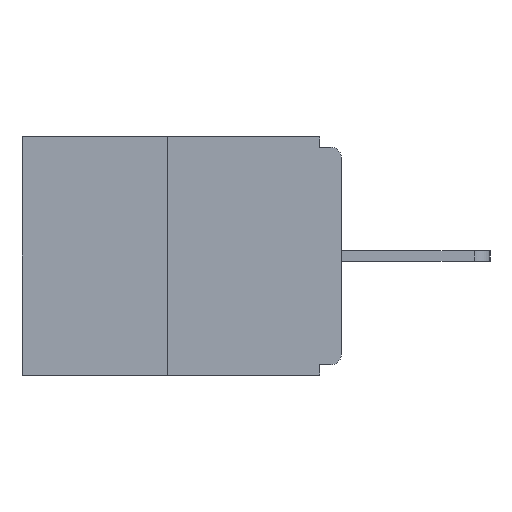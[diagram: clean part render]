
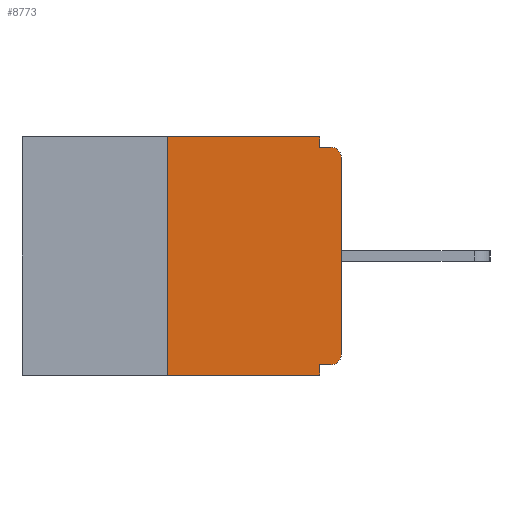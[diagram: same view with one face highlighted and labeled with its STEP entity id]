
A CAD part, left-side view. The second image highlights one B-rep face of the part: STEP entity #8773.
In plain terms, the highlighted planar face has unit normal (-1, 0, 0).
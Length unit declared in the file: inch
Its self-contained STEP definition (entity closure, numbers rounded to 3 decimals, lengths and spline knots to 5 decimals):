
#11 = DIRECTION ( 'NONE',  ( 0., 0., -1. ) ) ;
#30 = ORIENTED_EDGE ( 'NONE', *, *, #8550, .F. ) ;
#143 = VERTEX_POINT ( 'NONE', #796 ) ;
#256 = LINE ( 'NONE', #2933, #3321 ) ;
#281 = CARTESIAN_POINT ( 'NONE',  ( 0., 0.015, -0.03 ) ) ;
#344 = VERTEX_POINT ( 'NONE', #7226 ) ;
#379 = EDGE_CURVE ( 'NONE', #6385, #344, #6468, .T. ) ;
#405 = CARTESIAN_POINT ( 'NONE',  ( 0., 0.25, 0. ) ) ;
#621 = CARTESIAN_POINT ( 'NONE',  ( 0., 0.015, -0.313 ) ) ;
#660 = ORIENTED_EDGE ( 'NONE', *, *, #8884, .T. ) ;
#753 = CARTESIAN_POINT ( 'NONE',  ( 0., 0., -0.015 ) ) ;
#796 = CARTESIAN_POINT ( 'NONE',  ( 0., 0., -0.03 ) ) ;
#805 = EDGE_CURVE ( 'NONE', #2857, #3706, #3676, .T. ) ;
#1231 = CARTESIAN_POINT ( 'NONE',  ( 0., 0.031, -0.343 ) ) ;
#1601 = LINE ( 'NONE', #7221, #7797 ) ;
#1627 = VERTEX_POINT ( 'NONE', #2235 ) ;
#2040 = CARTESIAN_POINT ( 'NONE',  ( 0., 0.015, -0.015 ) ) ;
#2138 = PLANE ( 'NONE',  #8941 ) ;
#2140 = CARTESIAN_POINT ( 'NONE',  ( 0., 0.25, -0.343 ) ) ;
#2206 = CARTESIAN_POINT ( 'NONE',  ( 0., 0.25, 0. ) ) ;
#2216 = ORIENTED_EDGE ( 'NONE', *, *, #3671, .F. ) ;
#2235 = CARTESIAN_POINT ( 'NONE',  ( 0., 0.031, 0. ) ) ;
#2557 = DIRECTION ( 'NONE',  ( 0., -1., 0. ) ) ;
#2826 = DIRECTION ( 'NONE',  ( 0., 0., 1. ) ) ;
#2857 = VERTEX_POINT ( 'NONE', #2140 ) ;
#2933 = CARTESIAN_POINT ( 'NONE',  ( 0., 0.46, 0. ) ) ;
#3038 = VECTOR ( 'NONE', #10724, 39.37008 ) ;
#3268 = VECTOR ( 'NONE', #11126, 39.37008 ) ;
#3321 = VECTOR ( 'NONE', #9199, 39.37008 ) ;
#3358 = CARTESIAN_POINT ( 'NONE',  ( 0., 0., -0.313 ) ) ;
#3641 = CARTESIAN_POINT ( 'NONE',  ( 0., 0., -0.328 ) ) ;
#3671 = EDGE_CURVE ( 'NONE', #9577, #1627, #256, .T. ) ;
#3676 = LINE ( 'NONE', #7213, #3038 ) ;
#3706 = VERTEX_POINT ( 'NONE', #1231 ) ;
#3838 = ORIENTED_EDGE ( 'NONE', *, *, #6048, .T. ) ;
#3897 = CARTESIAN_POINT ( 'NONE',  ( 0., 0.031, -0.015 ) ) ;
#3937 = FACE_OUTER_BOUND ( 'NONE', #4985, .T. ) ;
#4166 = VERTEX_POINT ( 'NONE', #3358 ) ;
#4180 = DIRECTION ( 'NONE',  ( -1., 0., 0. ) ) ;
#4851 = CARTESIAN_POINT ( 'NONE',  ( 0., 0.015, -0.328 ) ) ;
#4985 = EDGE_LOOP ( 'NONE', ( #2216, #7420, #8990, #8470, #5005, #660, #3838, #9968, #30, #7469 ) ) ;
#5005 = ORIENTED_EDGE ( 'NONE', *, *, #379, .F. ) ;
#5218 = AXIS2_PLACEMENT_3D ( 'NONE', #281, #6819, #9435 ) ;
#5239 = EDGE_CURVE ( 'NONE', #1627, #11204, #9710, .T. ) ;
#5415 = VERTEX_POINT ( 'NONE', #2040 ) ;
#5509 = EDGE_CURVE ( 'NONE', #2857, #9577, #7735, .T. ) ;
#5727 = CARTESIAN_POINT ( 'NONE',  ( 0., 0.46, 0. ) ) ;
#6048 = EDGE_CURVE ( 'NONE', #4166, #143, #1601, .T. ) ;
#6277 = CARTESIAN_POINT ( 'NONE',  ( 0., 0.031, 0. ) ) ;
#6385 = VERTEX_POINT ( 'NONE', #4851 ) ;
#6458 = VECTOR ( 'NONE', #11, 39.37008 ) ;
#6468 = LINE ( 'NONE', #3641, #11161 ) ;
#6523 = VECTOR ( 'NONE', #2557, 39.37008 ) ;
#6658 = DIRECTION ( 'NONE',  ( 1., 0., 0. ) ) ;
#6726 = AXIS2_PLACEMENT_3D ( 'NONE', #621, #4180, #8639 ) ;
#6819 = DIRECTION ( 'NONE',  ( -1., 0., 0. ) ) ;
#6977 = LINE ( 'NONE', #11251, #9116 ) ;
#7170 = DIRECTION ( 'NONE',  ( 0., 1., 0. ) ) ;
#7213 = CARTESIAN_POINT ( 'NONE',  ( 0., 0.46, -0.343 ) ) ;
#7221 = CARTESIAN_POINT ( 'NONE',  ( 0., 0., 0. ) ) ;
#7226 = CARTESIAN_POINT ( 'NONE',  ( 0., 0.031, -0.328 ) ) ;
#7420 = ORIENTED_EDGE ( 'NONE', *, *, #5509, .F. ) ;
#7469 = ORIENTED_EDGE ( 'NONE', *, *, #5239, .F. ) ;
#7618 = EDGE_CURVE ( 'NONE', #143, #5415, #10922, .T. ) ;
#7735 = LINE ( 'NONE', #2206, #3268 ) ;
#7797 = VECTOR ( 'NONE', #2826, 39.37008 ) ;
#8209 = EDGE_CURVE ( 'NONE', #344, #3706, #6977, .T. ) ;
#8470 = ORIENTED_EDGE ( 'NONE', *, *, #8209, .F. ) ;
#8550 = EDGE_CURVE ( 'NONE', #11204, #5415, #8763, .T. ) ;
#8639 = DIRECTION ( 'NONE',  ( 0., 0., -1. ) ) ;
#8763 = LINE ( 'NONE', #753, #6523 ) ;
#8773 = ADVANCED_FACE ( 'NONE', ( #3937 ), #2138, .F. ) ;
#8884 = EDGE_CURVE ( 'NONE', #6385, #4166, #9864, .T. ) ;
#8941 = AXIS2_PLACEMENT_3D ( 'NONE', #5727, #6658, #10193 ) ;
#8990 = ORIENTED_EDGE ( 'NONE', *, *, #805, .T. ) ;
#9116 = VECTOR ( 'NONE', #10497, 39.37008 ) ;
#9199 = DIRECTION ( 'NONE',  ( 0., -1., 0. ) ) ;
#9435 = DIRECTION ( 'NONE',  ( 0., 0., -1. ) ) ;
#9577 = VERTEX_POINT ( 'NONE', #405 ) ;
#9710 = LINE ( 'NONE', #6277, #6458 ) ;
#9864 = CIRCLE ( 'NONE', #6726, 0.015 ) ;
#9968 = ORIENTED_EDGE ( 'NONE', *, *, #7618, .T. ) ;
#10193 = DIRECTION ( 'NONE',  ( 0., 0., -1. ) ) ;
#10497 = DIRECTION ( 'NONE',  ( 0., 0., -1. ) ) ;
#10724 = DIRECTION ( 'NONE',  ( 0., -1., 0. ) ) ;
#10922 = CIRCLE ( 'NONE', #5218, 0.015 ) ;
#11126 = DIRECTION ( 'NONE',  ( 0., 0., 1. ) ) ;
#11161 = VECTOR ( 'NONE', #7170, 39.37008 ) ;
#11204 = VERTEX_POINT ( 'NONE', #3897 ) ;
#11251 = CARTESIAN_POINT ( 'NONE',  ( 0., 0.031, -0.343 ) ) ;
